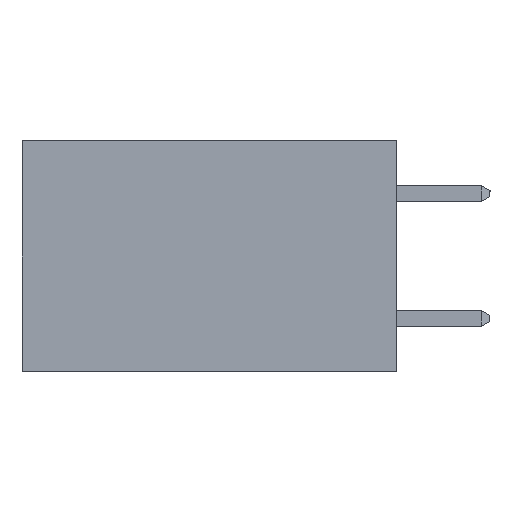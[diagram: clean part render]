
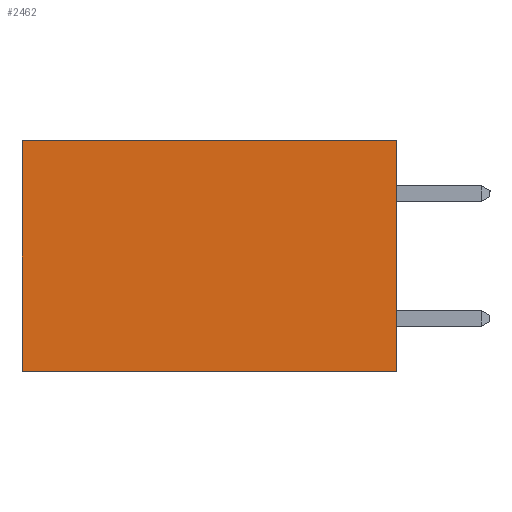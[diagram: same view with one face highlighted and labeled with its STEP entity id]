
A CAD part, left-side view. The second image highlights one B-rep face of the part: STEP entity #2462.
In plain terms, the highlighted planar face has unit normal (-1, 0, 0).
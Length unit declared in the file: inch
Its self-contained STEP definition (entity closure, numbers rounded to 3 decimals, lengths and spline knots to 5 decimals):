
#121 = EDGE_CURVE ( 'NONE', #7858, #7257, #11377, .T. ) ;
#323 = VECTOR ( 'NONE', #3032, 39.37008 ) ;
#423 = CARTESIAN_POINT ( 'NONE',  ( 0.2615, 0., -0.37 ) ) ;
#1168 = VERTEX_POINT ( 'NONE', #2305 ) ;
#1450 = CARTESIAN_POINT ( 'NONE',  ( 0.2615, 0., -0.37 ) ) ;
#2305 = CARTESIAN_POINT ( 'NONE',  ( 0.2615, 0.6, 0. ) ) ;
#2462 = ADVANCED_FACE ( 'NONE', ( #5653 ), #4736, .F. ) ;
#3032 = DIRECTION ( 'NONE',  ( 0., 0., -1. ) ) ;
#3229 = EDGE_CURVE ( 'NONE', #7522, #7858, #3767, .T. ) ;
#3676 = AXIS2_PLACEMENT_3D ( 'NONE', #3749, #12247, #9086 ) ;
#3749 = CARTESIAN_POINT ( 'NONE',  ( 0.2615, 0., -0.37 ) ) ;
#3767 = LINE ( 'NONE', #423, #6194 ) ;
#4003 = CARTESIAN_POINT ( 'NONE',  ( 0.2615, 0., 0. ) ) ;
#4385 = EDGE_CURVE ( 'NONE', #1168, #7257, #9287, .T. ) ;
#4736 = PLANE ( 'NONE',  #3676 ) ;
#4959 = CARTESIAN_POINT ( 'NONE',  ( 0.2615, 0., 0. ) ) ;
#5099 = ORIENTED_EDGE ( 'NONE', *, *, #13684, .T. ) ;
#5268 = DIRECTION ( 'NONE',  ( 0., 1., 0. ) ) ;
#5653 = FACE_OUTER_BOUND ( 'NONE', #6309, .T. ) ;
#6194 = VECTOR ( 'NONE', #11058, 39.37008 ) ;
#6309 = EDGE_LOOP ( 'NONE', ( #9498, #11029, #8588, #5099 ) ) ;
#7257 = VERTEX_POINT ( 'NONE', #13084 ) ;
#7522 = VERTEX_POINT ( 'NONE', #4003 ) ;
#7858 = VERTEX_POINT ( 'NONE', #1450 ) ;
#8588 = ORIENTED_EDGE ( 'NONE', *, *, #3229, .F. ) ;
#9086 = DIRECTION ( 'NONE',  ( 0., 0., -1. ) ) ;
#9287 = LINE ( 'NONE', #12663, #323 ) ;
#9498 = ORIENTED_EDGE ( 'NONE', *, *, #4385, .T. ) ;
#9555 = DIRECTION ( 'NONE',  ( 0., 1., 0. ) ) ;
#9690 = VECTOR ( 'NONE', #9555, 39.37008 ) ;
#10326 = CARTESIAN_POINT ( 'NONE',  ( 0.2615, 0., -0.37 ) ) ;
#11029 = ORIENTED_EDGE ( 'NONE', *, *, #121, .F. ) ;
#11058 = DIRECTION ( 'NONE',  ( 0., 0., -1. ) ) ;
#11377 = LINE ( 'NONE', #10326, #11957 ) ;
#11957 = VECTOR ( 'NONE', #5268, 39.37008 ) ;
#12247 = DIRECTION ( 'NONE',  ( 1., 0., 0. ) ) ;
#12663 = CARTESIAN_POINT ( 'NONE',  ( 0.2615, 0.6, -0.37 ) ) ;
#13084 = CARTESIAN_POINT ( 'NONE',  ( 0.2615, 0.6, -0.37 ) ) ;
#13455 = LINE ( 'NONE', #4959, #9690 ) ;
#13684 = EDGE_CURVE ( 'NONE', #7522, #1168, #13455, .T. ) ;
